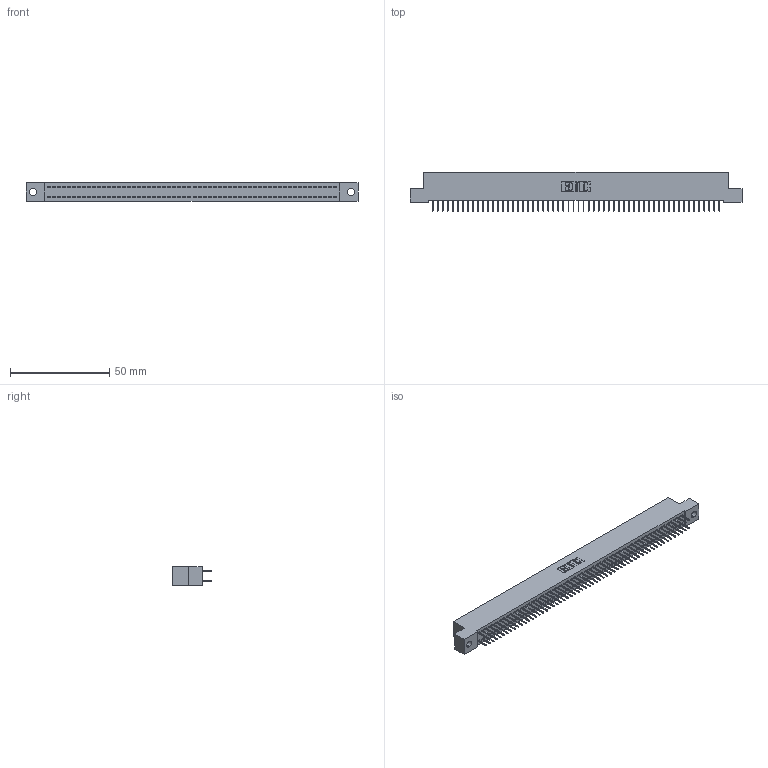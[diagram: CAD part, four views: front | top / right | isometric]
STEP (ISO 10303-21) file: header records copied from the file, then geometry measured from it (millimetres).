
FILE_DESCRIPTION (( 'STEP AP203' ), '1' );
FILE_NAME ('342-116-524-202.STEP', '2018-08-14T13:33:17', ( '' ), ( '' ), 'SwSTEP 2.0', 'SolidWorks 2016', '' );
FILE_SCHEMA (( 'CONFIG_CONTROL_DESIGN' ));
Length unit declared in the file: inch
Products named in the file (3): 342-116-524-202; 342 Part_.128 Slot; 345-292-001_345-293-124
Assembly tree (117 placements, depth 2):
  342-116-524-202
    342 Part_.128 Slot
    345-292-001_345-293-124  x116
Bounding box: 167.64 x 19.69 x 9.4 mm (x, y, z)
Volume: 14910.5 mm3; surface area: 23967.6 mm2
Topology: 117 solids, 117 shells, 6610 faces, 18755 edges, 12038 vertices
Faces by surface type: plane 4942, cylinder 1668
Entity records: 35321 total; most frequent: CARTESIAN_POINT 5834, ORIENTED_EDGE 5770, DIRECTION 4957, EDGE_CURVE 2885, VECTOR 2761, LINE 2761, VERTEX_POINT 1918, AXIS2_PLACEMENT_3D 1098
